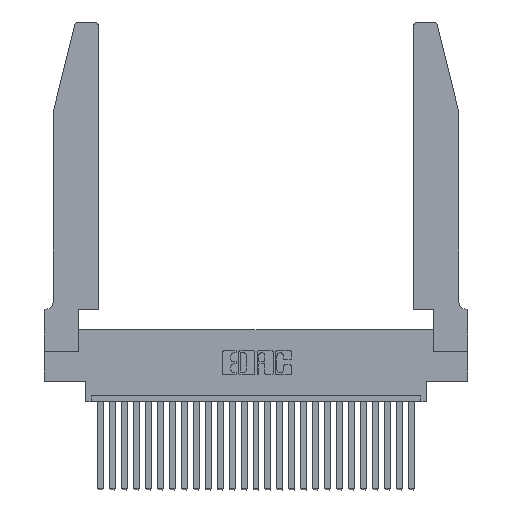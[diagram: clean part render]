
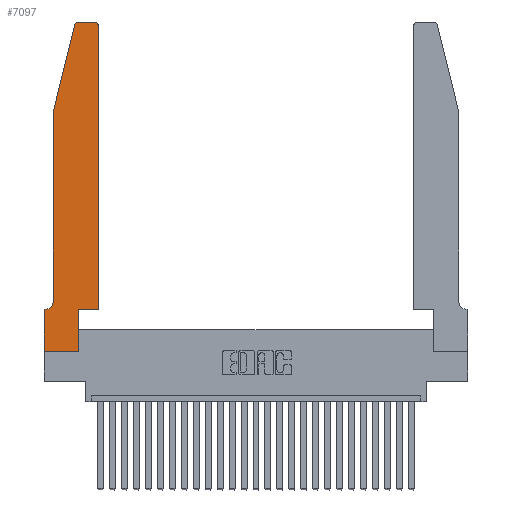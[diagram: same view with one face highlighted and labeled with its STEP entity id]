
A CAD part, top view. The second image highlights one B-rep face of the part: STEP entity #7097.
In plain terms, the highlighted planar face has unit normal (0, 0, 1).
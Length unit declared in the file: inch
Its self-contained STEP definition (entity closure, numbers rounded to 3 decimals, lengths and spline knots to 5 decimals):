
#341 = VECTOR ( 'NONE', #25861, 39.37008 ) ;
#415 = CARTESIAN_POINT ( 'NONE',  ( 0.25487, 2.72718, 0.37 ) ) ;
#584 = ORIENTED_EDGE ( 'NONE', *, *, #16813, .T. ) ;
#653 = DIRECTION ( 'NONE',  ( 1., 0., 0. ) ) ;
#782 = CARTESIAN_POINT ( 'NONE',  ( 0.2865, 0.35, 0.37 ) ) ;
#1103 = VECTOR ( 'NONE', #21884, 39.37008 ) ;
#1314 = VERTEX_POINT ( 'NONE', #16141 ) ;
#2284 = ORIENTED_EDGE ( 'NONE', *, *, #18637, .T. ) ;
#2453 = VECTOR ( 'NONE', #19846, 39.37008 ) ;
#3024 = VERTEX_POINT ( 'NONE', #13901 ) ;
#3070 = ORIENTED_EDGE ( 'NONE', *, *, #15990, .T. ) ;
#3138 = VECTOR ( 'NONE', #19694, 39.37008 ) ;
#3342 = DIRECTION ( 'NONE',  ( 0., -1., 0. ) ) ;
#4814 = DIRECTION ( 'NONE',  ( 1., 0., 0. ) ) ;
#5086 = CARTESIAN_POINT ( 'NONE',  ( 0., 0., 0.37 ) ) ;
#5349 = VECTOR ( 'NONE', #7571, 39.37008 ) ;
#5444 = CARTESIAN_POINT ( 'NONE',  ( 0.0755, 2., 0.37 ) ) ;
#5928 = VERTEX_POINT ( 'NONE', #20348 ) ;
#6107 = CARTESIAN_POINT ( 'NONE',  ( 0.0755, 0.42, 0.37 ) ) ;
#6307 = CARTESIAN_POINT ( 'NONE',  ( 0., 0., 0.37 ) ) ;
#6723 = LINE ( 'NONE', #782, #1103 ) ;
#6762 = VERTEX_POINT ( 'NONE', #6307 ) ;
#7097 = ADVANCED_FACE ( 'NONE', ( #11607 ), #16939, .T. ) ;
#7151 = EDGE_CURVE ( 'NONE', #5928, #16380, #6723, .T. ) ;
#7275 = EDGE_CURVE ( 'NONE', #16380, #15851, #7395, .T. ) ;
#7395 = LINE ( 'NONE', #21680, #2453 ) ;
#7550 = DIRECTION ( 'NONE',  ( 0., 0., 1. ) ) ;
#7571 = DIRECTION ( 'NONE',  ( -0.239, -0.971, 0. ) ) ;
#7648 = LINE ( 'NONE', #5444, #5349 ) ;
#7889 = AXIS2_PLACEMENT_3D ( 'NONE', #26003, #17608, #4814 ) ;
#8064 = DIRECTION ( 'NONE',  ( 1., 0., 0. ) ) ;
#8451 = EDGE_CURVE ( 'NONE', #6762, #5928, #11923, .T. ) ;
#8456 = CARTESIAN_POINT ( 'NONE',  ( 0.4505, 0.35, 0.37 ) ) ;
#8710 = CIRCLE ( 'NONE', #20492, 0.07 ) ;
#8982 = VECTOR ( 'NONE', #8064, 39.37008 ) ;
#9281 = VECTOR ( 'NONE', #3342, 39.37008 ) ;
#9307 = CARTESIAN_POINT ( 'NONE',  ( 0.0755, 2., 0.37 ) ) ;
#9366 = DIRECTION ( 'NONE',  ( 0., 0., 1. ) ) ;
#9593 = LINE ( 'NONE', #9307, #9281 ) ;
#9651 = ORIENTED_EDGE ( 'NONE', *, *, #26418, .T. ) ;
#9789 = VERTEX_POINT ( 'NONE', #14722 ) ;
#10520 = CARTESIAN_POINT ( 'NONE',  ( 0.4505, 2.72, 0.37 ) ) ;
#10825 = ORIENTED_EDGE ( 'NONE', *, *, #15503, .T. ) ;
#11183 = CARTESIAN_POINT ( 'NONE',  ( 0.4505, 0.35, 0.37 ) ) ;
#11607 = FACE_OUTER_BOUND ( 'NONE', #14865, .T. ) ;
#11656 = DIRECTION ( 'NONE',  ( 1., 0., 0. ) ) ;
#11923 = LINE ( 'NONE', #14009, #8982 ) ;
#12289 = VECTOR ( 'NONE', #21690, 39.37008 ) ;
#12411 = ORIENTED_EDGE ( 'NONE', *, *, #16969, .T. ) ;
#12841 = DIRECTION ( 'NONE',  ( 0., 1., 0. ) ) ;
#12865 = ORIENTED_EDGE ( 'NONE', *, *, #8451, .T. ) ;
#12917 = CIRCLE ( 'NONE', #17542, 0.03 ) ;
#13419 = VERTEX_POINT ( 'NONE', #415 ) ;
#13584 = EDGE_CURVE ( 'NONE', #9789, #16280, #26641, .T. ) ;
#13633 = LINE ( 'NONE', #5086, #3138 ) ;
#13901 = CARTESIAN_POINT ( 'NONE',  ( 0.0755, 2., 0.37 ) ) ;
#14009 = CARTESIAN_POINT ( 'NONE',  ( 0., 0., 0.37 ) ) ;
#14722 = CARTESIAN_POINT ( 'NONE',  ( 0.0055, 0.35, 0.37 ) ) ;
#14865 = EDGE_LOOP ( 'NONE', ( #2284, #10825, #12411, #17961, #3070, #21835, #9651, #12865, #19688, #15149, #26840, #584 ) ) ;
#14952 = CIRCLE ( 'NONE', #24713, 0.03 ) ;
#15149 = ORIENTED_EDGE ( 'NONE', *, *, #7275, .T. ) ;
#15503 = EDGE_CURVE ( 'NONE', #1314, #13419, #14952, .T. ) ;
#15579 = CARTESIAN_POINT ( 'NONE',  ( 0.4205, 2.72, 0.37 ) ) ;
#15593 = CARTESIAN_POINT ( 'NONE',  ( 0.0055, 0.42, 0.37 ) ) ;
#15723 = EDGE_CURVE ( 'NONE', #15851, #18777, #17206, .T. ) ;
#15851 = VERTEX_POINT ( 'NONE', #11183 ) ;
#15990 = EDGE_CURVE ( 'NONE', #18388, #9789, #8710, .T. ) ;
#16141 = CARTESIAN_POINT ( 'NONE',  ( 0.284, 2.75, 0.37 ) ) ;
#16280 = VERTEX_POINT ( 'NONE', #24891 ) ;
#16380 = VERTEX_POINT ( 'NONE', #18770 ) ;
#16813 = EDGE_CURVE ( 'NONE', #18777, #23241, #12917, .T. ) ;
#16939 = PLANE ( 'NONE',  #7889 ) ;
#16969 = EDGE_CURVE ( 'NONE', #13419, #3024, #7648, .T. ) ;
#17206 = LINE ( 'NONE', #8456, #25701 ) ;
#17467 = CARTESIAN_POINT ( 'NONE',  ( 0.2605, 2.75, 0.37 ) ) ;
#17542 = AXIS2_PLACEMENT_3D ( 'NONE', #15579, #9366, #653 ) ;
#17608 = DIRECTION ( 'NONE',  ( 0., 0., 1. ) ) ;
#17961 = ORIENTED_EDGE ( 'NONE', *, *, #21934, .T. ) ;
#18388 = VERTEX_POINT ( 'NONE', #6107 ) ;
#18637 = EDGE_CURVE ( 'NONE', #23241, #1314, #23901, .T. ) ;
#18770 = CARTESIAN_POINT ( 'NONE',  ( 0.2865, 0.35, 0.37 ) ) ;
#18777 = VERTEX_POINT ( 'NONE', #10520 ) ;
#19296 = DIRECTION ( 'NONE',  ( 0., 0., -1. ) ) ;
#19688 = ORIENTED_EDGE ( 'NONE', *, *, #7151, .T. ) ;
#19694 = DIRECTION ( 'NONE',  ( 0., -1., 0. ) ) ;
#19846 = DIRECTION ( 'NONE',  ( 1., 0., 0. ) ) ;
#20348 = CARTESIAN_POINT ( 'NONE',  ( 0.2865, 0., 0.37 ) ) ;
#20478 = CARTESIAN_POINT ( 'NONE',  ( 0.4205, 2.75, 0.37 ) ) ;
#20492 = AXIS2_PLACEMENT_3D ( 'NONE', #15593, #19296, #22583 ) ;
#21680 = CARTESIAN_POINT ( 'NONE',  ( 0.4505, 0.35, 0.37 ) ) ;
#21690 = DIRECTION ( 'NONE',  ( -1., 0., 0. ) ) ;
#21835 = ORIENTED_EDGE ( 'NONE', *, *, #13584, .T. ) ;
#21884 = DIRECTION ( 'NONE',  ( 0., 1., 0. ) ) ;
#21934 = EDGE_CURVE ( 'NONE', #3024, #18388, #9593, .T. ) ;
#22051 = CARTESIAN_POINT ( 'NONE',  ( 0.0755, 0.35, 0.37 ) ) ;
#22583 = DIRECTION ( 'NONE',  ( -1., 0., 0. ) ) ;
#23241 = VERTEX_POINT ( 'NONE', #20478 ) ;
#23901 = LINE ( 'NONE', #17467, #341 ) ;
#24164 = CARTESIAN_POINT ( 'NONE',  ( 0.284, 2.72, 0.37 ) ) ;
#24713 = AXIS2_PLACEMENT_3D ( 'NONE', #24164, #7550, #11656 ) ;
#24891 = CARTESIAN_POINT ( 'NONE',  ( 0., 0.35, 0.37 ) ) ;
#25701 = VECTOR ( 'NONE', #12841, 39.37008 ) ;
#25861 = DIRECTION ( 'NONE',  ( -1., 0., 0. ) ) ;
#26003 = CARTESIAN_POINT ( 'NONE',  ( 0., 0.35, 0.37 ) ) ;
#26418 = EDGE_CURVE ( 'NONE', #16280, #6762, #13633, .T. ) ;
#26641 = LINE ( 'NONE', #22051, #12289 ) ;
#26840 = ORIENTED_EDGE ( 'NONE', *, *, #15723, .T. ) ;
